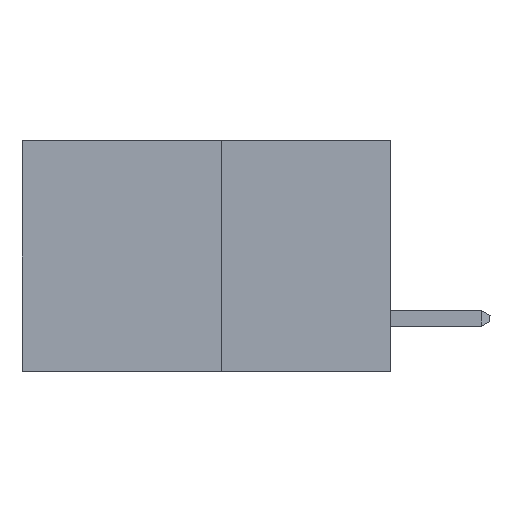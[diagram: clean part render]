
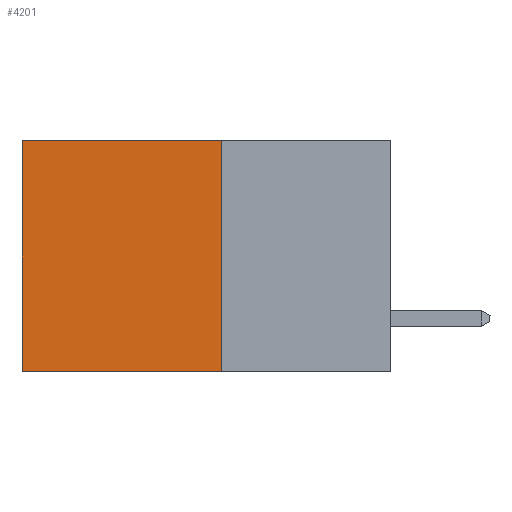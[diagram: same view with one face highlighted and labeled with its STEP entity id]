
A CAD part, left-side view. The second image highlights one B-rep face of the part: STEP entity #4201.
In plain terms, the highlighted planar face has unit normal (-1, 0, 0).
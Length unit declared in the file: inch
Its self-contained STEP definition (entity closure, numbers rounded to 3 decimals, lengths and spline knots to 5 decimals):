
#3 = PLANE ( 'NONE',  #1843 ) ;
#22 = CARTESIAN_POINT ( 'NONE',  ( 0.277, 0.27, 0. ) ) ;
#45 = EDGE_CURVE ( 'NONE', #232, #5156, #4556, .T. ) ;
#232 = VERTEX_POINT ( 'NONE', #6751 ) ;
#382 = DIRECTION ( 'NONE',  ( 0., 0., -1. ) ) ;
#517 = VECTOR ( 'NONE', #5814, 39.37008 ) ;
#854 = VECTOR ( 'NONE', #7799, 39.37008 ) ;
#1244 = CARTESIAN_POINT ( 'NONE',  ( 0.277, 0.59, -0.37 ) ) ;
#1406 = VECTOR ( 'NONE', #4163, 39.37008 ) ;
#1454 = VECTOR ( 'NONE', #382, 39.37008 ) ;
#1483 = DIRECTION ( 'NONE',  ( 0., 0., -1. ) ) ;
#1542 = VERTEX_POINT ( 'NONE', #6667 ) ;
#1557 = CARTESIAN_POINT ( 'NONE',  ( 0.277, 0.27, -0.37 ) ) ;
#1639 = ORIENTED_EDGE ( 'NONE', *, *, #45, .T. ) ;
#1698 = LINE ( 'NONE', #5583, #1454 ) ;
#1843 = AXIS2_PLACEMENT_3D ( 'NONE', #1557, #1932, #1483 ) ;
#1932 = DIRECTION ( 'NONE',  ( 1., 0., 0. ) ) ;
#2661 = CARTESIAN_POINT ( 'NONE',  ( 0.277, 0.59, -0.37 ) ) ;
#2708 = EDGE_CURVE ( 'NONE', #6788, #232, #3422, .T. ) ;
#3074 = ORIENTED_EDGE ( 'NONE', *, *, #8932, .F. ) ;
#3422 = LINE ( 'NONE', #5820, #1406 ) ;
#3546 = CARTESIAN_POINT ( 'NONE',  ( 0.277, 0.27, -0.37 ) ) ;
#4163 = DIRECTION ( 'NONE',  ( 0., 1., 0. ) ) ;
#4201 = ADVANCED_FACE ( 'NONE', ( #8286 ), #3, .F. ) ;
#4556 = LINE ( 'NONE', #2661, #517 ) ;
#5156 = VERTEX_POINT ( 'NONE', #1244 ) ;
#5583 = CARTESIAN_POINT ( 'NONE',  ( 0.277, 0.27, -0.37 ) ) ;
#5804 = EDGE_LOOP ( 'NONE', ( #1639, #3074, #8745, #8975 ) ) ;
#5814 = DIRECTION ( 'NONE',  ( 0., 0., -1. ) ) ;
#5820 = CARTESIAN_POINT ( 'NONE',  ( 0.277, 0.27, 0. ) ) ;
#6425 = EDGE_CURVE ( 'NONE', #6788, #1542, #1698, .T. ) ;
#6667 = CARTESIAN_POINT ( 'NONE',  ( 0.277, 0.27, -0.37 ) ) ;
#6751 = CARTESIAN_POINT ( 'NONE',  ( 0.277, 0.59, 0. ) ) ;
#6788 = VERTEX_POINT ( 'NONE', #22 ) ;
#6922 = LINE ( 'NONE', #3546, #854 ) ;
#7799 = DIRECTION ( 'NONE',  ( 0., 1., 0. ) ) ;
#8286 = FACE_OUTER_BOUND ( 'NONE', #5804, .T. ) ;
#8745 = ORIENTED_EDGE ( 'NONE', *, *, #6425, .F. ) ;
#8932 = EDGE_CURVE ( 'NONE', #1542, #5156, #6922, .T. ) ;
#8975 = ORIENTED_EDGE ( 'NONE', *, *, #2708, .T. ) ;
